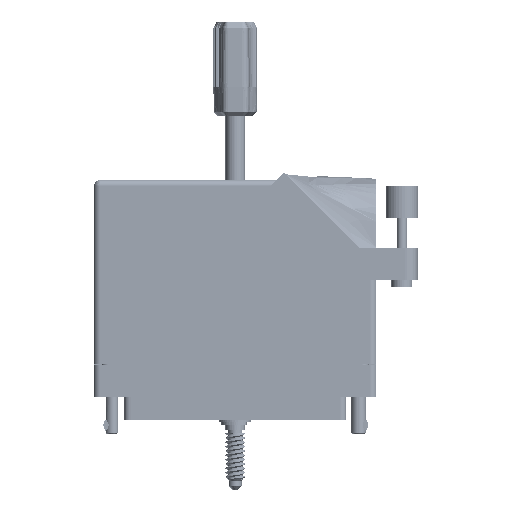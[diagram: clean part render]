
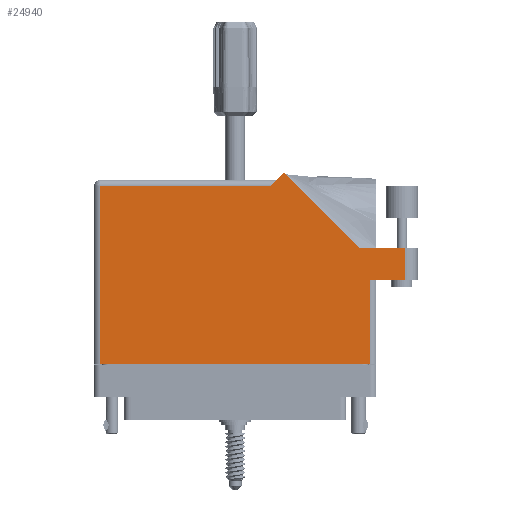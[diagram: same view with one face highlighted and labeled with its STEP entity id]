
A CAD part, front view. The second image highlights one B-rep face of the part: STEP entity #24940.
In plain terms, the highlighted face is planar.
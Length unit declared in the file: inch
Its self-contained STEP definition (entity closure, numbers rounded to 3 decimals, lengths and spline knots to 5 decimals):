
#119 = ORIENTED_EDGE ( 'NONE', *, *, #40146, .T. ) ;
#4110 = EDGE_CURVE ( 'NONE', #63360, #60250, #74733, .T. ) ;
#7740 = LINE ( 'NONE', #91507, #10061 ) ;
#10061 = VECTOR ( 'NONE', #69285, 39.37008 ) ;
#10236 = CARTESIAN_POINT ( 'NONE',  ( 0.337, 1.613, 0.617 ) ) ;
#12104 = DIRECTION ( 'NONE',  ( 0., 0., -1. ) ) ;
#13757 = LINE ( 'NONE', #80204, #91061 ) ;
#14431 = LINE ( 'NONE', #43409, #91726 ) ;
#14773 = LINE ( 'NONE', #18776, #81596 ) ;
#17606 = DIRECTION ( 'NONE',  ( -0.707, 0.707, 0. ) ) ;
#18776 = CARTESIAN_POINT ( 'NONE',  ( -1.359, -0.1, 0.617 ) ) ;
#21989 = EDGE_CURVE ( 'NONE', #89549, #34909, #49716, .T. ) ;
#22632 = EDGE_LOOP ( 'NONE', ( #36465, #80690, #25309, #42621, #28614, #119, #52927, #31603, #65916 ) ) ;
#22700 = CARTESIAN_POINT ( 'NONE',  ( 0.46971, 1.74571, 0.617 ) ) ;
#24940 = ADVANCED_FACE ( 'NONE', ( #38081 ), #63571, .F. ) ;
#25226 = DIRECTION ( 'NONE',  ( -0.707, -0.707, 0. ) ) ;
#25309 = ORIENTED_EDGE ( 'NONE', *, *, #42488, .T. ) ;
#25413 = CARTESIAN_POINT ( 'NONE',  ( 1.19342, 1.022, 0.617 ) ) ;
#28614 = ORIENTED_EDGE ( 'NONE', *, *, #37499, .T. ) ;
#28842 = EDGE_CURVE ( 'NONE', #88792, #48952, #50500, .T. ) ;
#30414 = CARTESIAN_POINT ( 'NONE',  ( 1.634, 0.715, 0.617 ) ) ;
#31603 = ORIENTED_EDGE ( 'NONE', *, *, #96056, .T. ) ;
#32838 = DIRECTION ( 'NONE',  ( 1., 0., 0. ) ) ;
#33658 = VECTOR ( 'NONE', #93536, 39.37008 ) ;
#34340 = CARTESIAN_POINT ( 'NONE',  ( -1.359, 1.675, 0.617 ) ) ;
#34909 = VERTEX_POINT ( 'NONE', #22700 ) ;
#36465 = ORIENTED_EDGE ( 'NONE', *, *, #91799, .T. ) ;
#37499 = EDGE_CURVE ( 'NONE', #34909, #84286, #52392, .T. ) ;
#38081 = FACE_OUTER_BOUND ( 'NONE', #22632, .T. ) ;
#38888 = CARTESIAN_POINT ( 'NONE',  ( -1.297, -0.1, 0.617 ) ) ;
#40146 = EDGE_CURVE ( 'NONE', #84286, #88792, #51203, .T. ) ;
#42339 = CARTESIAN_POINT ( 'NONE',  ( -1.297, -0.1, 0.617 ) ) ;
#42488 = EDGE_CURVE ( 'NONE', #60250, #89549, #7740, .T. ) ;
#42621 = ORIENTED_EDGE ( 'NONE', *, *, #21989, .T. ) ;
#43010 = VECTOR ( 'NONE', #45821, 39.37008 ) ;
#43409 = CARTESIAN_POINT ( 'NONE',  ( 1.359, 0.715, 0.617 ) ) ;
#43569 = CARTESIAN_POINT ( 'NONE',  ( -1.297, 1.613, 0.617 ) ) ;
#45821 = DIRECTION ( 'NONE',  ( 0., 1., 0. ) ) ;
#46011 = CARTESIAN_POINT ( 'NONE',  ( 1.634, 1.022, 0.617 ) ) ;
#48477 = CARTESIAN_POINT ( 'NONE',  ( 0.399, 1.675, 0.617 ) ) ;
#48952 = VERTEX_POINT ( 'NONE', #42339 ) ;
#49336 = CARTESIAN_POINT ( 'NONE',  ( -1.359, 1.613, 0.617 ) ) ;
#49716 = LINE ( 'NONE', #92224, #76689 ) ;
#50500 = LINE ( 'NONE', #38888, #59953 ) ;
#51203 = LINE ( 'NONE', #49336, #33658 ) ;
#52392 = LINE ( 'NONE', #48477, #61816 ) ;
#52927 = ORIENTED_EDGE ( 'NONE', *, *, #28842, .T. ) ;
#59585 = VERTEX_POINT ( 'NONE', #75629 ) ;
#59953 = VECTOR ( 'NONE', #69735, 39.37008 ) ;
#60250 = VERTEX_POINT ( 'NONE', #46011 ) ;
#61816 = VECTOR ( 'NONE', #25226, 39.37008 ) ;
#63360 = VERTEX_POINT ( 'NONE', #30414 ) ;
#63571 = PLANE ( 'NONE',  #95992 ) ;
#65916 = ORIENTED_EDGE ( 'NONE', *, *, #89105, .T. ) ;
#69285 = DIRECTION ( 'NONE',  ( -1., 0., 0. ) ) ;
#69735 = DIRECTION ( 'NONE',  ( 0., -1., 0. ) ) ;
#74733 = LINE ( 'NONE', #84103, #43010 ) ;
#75629 = CARTESIAN_POINT ( 'NONE',  ( 1.297, 0.715, 0.617 ) ) ;
#76689 = VECTOR ( 'NONE', #17606, 39.37008 ) ;
#80204 = CARTESIAN_POINT ( 'NONE',  ( 1.297, 0.715, 0.617 ) ) ;
#80690 = ORIENTED_EDGE ( 'NONE', *, *, #4110, .T. ) ;
#80757 = DIRECTION ( 'NONE',  ( 1., 0., 0. ) ) ;
#81074 = CARTESIAN_POINT ( 'NONE',  ( 1.297, -0.1, 0.617 ) ) ;
#81596 = VECTOR ( 'NONE', #32838, 39.37008 ) ;
#84103 = CARTESIAN_POINT ( 'NONE',  ( 1.634, 1.022, 0.617 ) ) ;
#84286 = VERTEX_POINT ( 'NONE', #10236 ) ;
#86752 = DIRECTION ( 'NONE',  ( -1., 0., 0. ) ) ;
#87074 = DIRECTION ( 'NONE',  ( 0., 1., 0. ) ) ;
#88792 = VERTEX_POINT ( 'NONE', #43569 ) ;
#89105 = EDGE_CURVE ( 'NONE', #91804, #59585, #13757, .T. ) ;
#89549 = VERTEX_POINT ( 'NONE', #25413 ) ;
#91061 = VECTOR ( 'NONE', #87074, 39.37008 ) ;
#91507 = CARTESIAN_POINT ( 'NONE',  ( 1.759, 1.022, 0.617 ) ) ;
#91726 = VECTOR ( 'NONE', #80757, 39.37008 ) ;
#91799 = EDGE_CURVE ( 'NONE', #59585, #63360, #14431, .T. ) ;
#91804 = VERTEX_POINT ( 'NONE', #81074 ) ;
#92224 = CARTESIAN_POINT ( 'NONE',  ( 1.19342, 1.022, 0.617 ) ) ;
#93536 = DIRECTION ( 'NONE',  ( -1., 0., 0. ) ) ;
#95992 = AXIS2_PLACEMENT_3D ( 'NONE', #34340, #12104, #86752 ) ;
#96056 = EDGE_CURVE ( 'NONE', #48952, #91804, #14773, .T. ) ;
